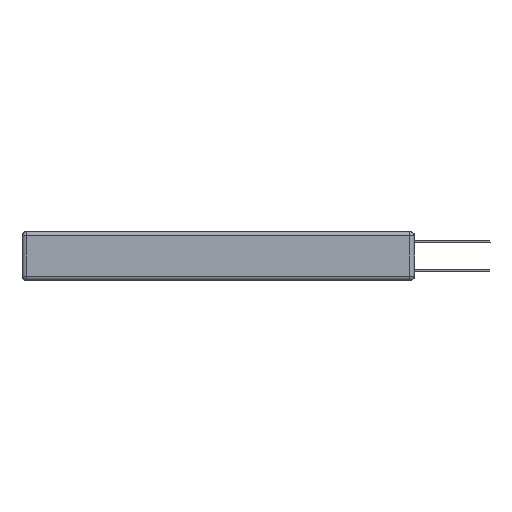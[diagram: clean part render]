
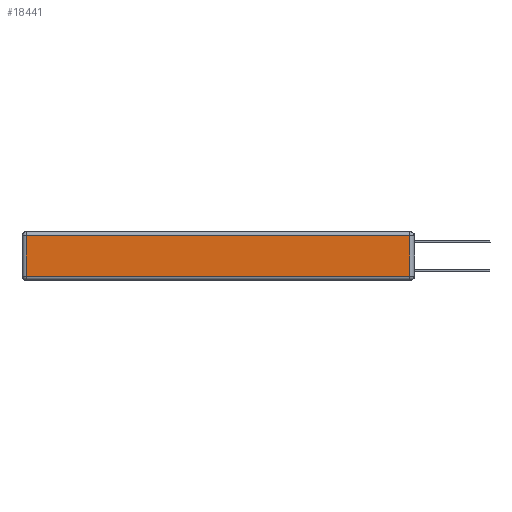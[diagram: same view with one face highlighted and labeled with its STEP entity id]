
A CAD part, left-side view. The second image highlights one B-rep face of the part: STEP entity #18441.
In plain terms, the highlighted planar face has unit normal (-1, 0, 0).
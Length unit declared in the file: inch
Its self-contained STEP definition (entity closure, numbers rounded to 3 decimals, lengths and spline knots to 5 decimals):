
#811 = VECTOR ( 'NONE', #11438, 39.37008 ) ;
#1104 = CARTESIAN_POINT ( 'NONE',  ( 0., 2.75, -0.03 ) ) ;
#1668 = VECTOR ( 'NONE', #12352, 39.37008 ) ;
#4561 = VERTEX_POINT ( 'NONE', #9559 ) ;
#4759 = CARTESIAN_POINT ( 'NONE',  ( 0., 0.03, -0.03 ) ) ;
#4861 = LINE ( 'NONE', #6128, #811 ) ;
#4976 = VERTEX_POINT ( 'NONE', #8858 ) ;
#5176 = EDGE_CURVE ( 'NONE', #4976, #5566, #4861, .T. ) ;
#5566 = VERTEX_POINT ( 'NONE', #17589 ) ;
#6128 = CARTESIAN_POINT ( 'NONE',  ( 0., 2.72, -0.343 ) ) ;
#6837 = DIRECTION ( 'NONE',  ( -1., 0., 0. ) ) ;
#8088 = LINE ( 'NONE', #22372, #12136 ) ;
#8858 = CARTESIAN_POINT ( 'NONE',  ( 0., 2.72, -0.03 ) ) ;
#8958 = DIRECTION ( 'NONE',  ( 0., 0., 1. ) ) ;
#9559 = CARTESIAN_POINT ( 'NONE',  ( 0., 0.03, -0.313 ) ) ;
#10468 = CARTESIAN_POINT ( 'NONE',  ( 0., 0., -0.343 ) ) ;
#11438 = DIRECTION ( 'NONE',  ( 0., 0., -1. ) ) ;
#12136 = VECTOR ( 'NONE', #22443, 39.37008 ) ;
#12352 = DIRECTION ( 'NONE',  ( 0., -1., 0. ) ) ;
#13045 = LINE ( 'NONE', #21027, #1668 ) ;
#13400 = ORIENTED_EDGE ( 'NONE', *, *, #15407, .T. ) ;
#13478 = LINE ( 'NONE', #1104, #22192 ) ;
#13766 = EDGE_CURVE ( 'NONE', #4561, #16640, #8088, .T. ) ;
#14038 = PLANE ( 'NONE',  #20993 ) ;
#15407 = EDGE_CURVE ( 'NONE', #5566, #4561, #13045, .T. ) ;
#16300 = DIRECTION ( 'NONE',  ( 0., 1., 0. ) ) ;
#16640 = VERTEX_POINT ( 'NONE', #4759 ) ;
#17185 = ORIENTED_EDGE ( 'NONE', *, *, #13766, .T. ) ;
#17589 = CARTESIAN_POINT ( 'NONE',  ( 0., 2.72, -0.313 ) ) ;
#18118 = ORIENTED_EDGE ( 'NONE', *, *, #5176, .T. ) ;
#18441 = ADVANCED_FACE ( 'NONE', ( #19041 ), #14038, .T. ) ;
#19041 = FACE_OUTER_BOUND ( 'NONE', #20550, .T. ) ;
#19866 = ORIENTED_EDGE ( 'NONE', *, *, #21475, .T. ) ;
#20550 = EDGE_LOOP ( 'NONE', ( #13400, #17185, #19866, #18118 ) ) ;
#20993 = AXIS2_PLACEMENT_3D ( 'NONE', #10468, #6837, #8958 ) ;
#21027 = CARTESIAN_POINT ( 'NONE',  ( 0., 0., -0.313 ) ) ;
#21475 = EDGE_CURVE ( 'NONE', #16640, #4976, #13478, .T. ) ;
#22192 = VECTOR ( 'NONE', #16300, 39.37008 ) ;
#22372 = CARTESIAN_POINT ( 'NONE',  ( 0., 0.03, -0.343 ) ) ;
#22443 = DIRECTION ( 'NONE',  ( 0., 0., 1. ) ) ;
